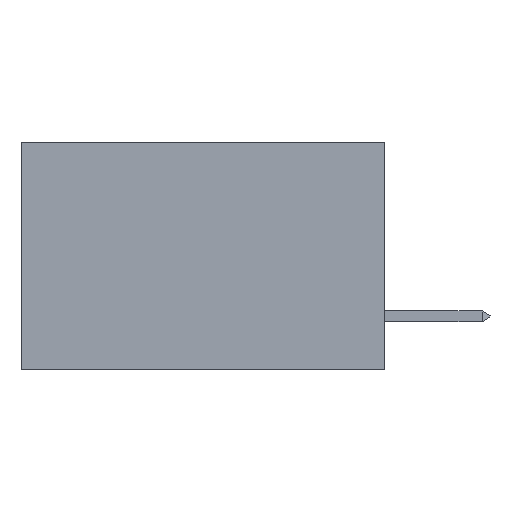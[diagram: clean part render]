
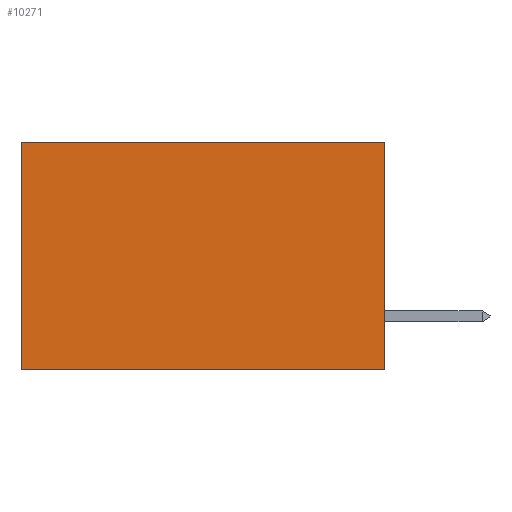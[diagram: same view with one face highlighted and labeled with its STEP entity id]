
A CAD part, left-side view. The second image highlights one B-rep face of the part: STEP entity #10271.
In plain terms, the highlighted planar face has unit normal (-1, 0, 0).
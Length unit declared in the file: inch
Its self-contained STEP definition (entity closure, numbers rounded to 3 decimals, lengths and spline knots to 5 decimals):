
#9 = VECTOR ( 'NONE', #11550, 39.37008 ) ;
#167 = DIRECTION ( 'NONE',  ( 1., 0., 0. ) ) ;
#1099 = AXIS2_PLACEMENT_3D ( 'NONE', #14096, #167, #14027 ) ;
#1627 = CARTESIAN_POINT ( 'NONE',  ( 0.2875, 0., -0.375 ) ) ;
#3702 = EDGE_CURVE ( 'NONE', #12875, #6642, #11055, .T. ) ;
#4436 = PLANE ( 'NONE',  #1099 ) ;
#5596 = CARTESIAN_POINT ( 'NONE',  ( 0.2875, 0.6, 0. ) ) ;
#5599 = LINE ( 'NONE', #14224, #12664 ) ;
#6515 = CARTESIAN_POINT ( 'NONE',  ( 0.2875, 0.6, -0.375 ) ) ;
#6580 = CARTESIAN_POINT ( 'NONE',  ( 0.2875, 0.6, -0.375 ) ) ;
#6642 = VERTEX_POINT ( 'NONE', #5596 ) ;
#7255 = ORIENTED_EDGE ( 'NONE', *, *, #12649, .F. ) ;
#7538 = VERTEX_POINT ( 'NONE', #1627 ) ;
#7686 = CARTESIAN_POINT ( 'NONE',  ( 0.2875, 0., 0. ) ) ;
#8364 = VERTEX_POINT ( 'NONE', #6580 ) ;
#8438 = EDGE_CURVE ( 'NONE', #6642, #8364, #12751, .T. ) ;
#9374 = CARTESIAN_POINT ( 'NONE',  ( 0.2875, 0., 0. ) ) ;
#9626 = EDGE_LOOP ( 'NONE', ( #13773, #7255, #12810, #14415 ) ) ;
#10271 = ADVANCED_FACE ( 'NONE', ( #15591 ), #4436, .F. ) ;
#11055 = LINE ( 'NONE', #9374, #15131 ) ;
#11550 = DIRECTION ( 'NONE',  ( 0., 1., 0. ) ) ;
#11990 = DIRECTION ( 'NONE',  ( 0., 1., 0. ) ) ;
#12649 = EDGE_CURVE ( 'NONE', #7538, #8364, #16769, .T. ) ;
#12664 = VECTOR ( 'NONE', #14164, 39.37008 ) ;
#12751 = LINE ( 'NONE', #6515, #13849 ) ;
#12810 = ORIENTED_EDGE ( 'NONE', *, *, #13257, .F. ) ;
#12875 = VERTEX_POINT ( 'NONE', #7686 ) ;
#13257 = EDGE_CURVE ( 'NONE', #12875, #7538, #5599, .T. ) ;
#13773 = ORIENTED_EDGE ( 'NONE', *, *, #8438, .T. ) ;
#13849 = VECTOR ( 'NONE', #16125, 39.37008 ) ;
#14027 = DIRECTION ( 'NONE',  ( 0., 0., -1. ) ) ;
#14096 = CARTESIAN_POINT ( 'NONE',  ( 0.2875, 0., -0.375 ) ) ;
#14164 = DIRECTION ( 'NONE',  ( 0., 0., -1. ) ) ;
#14224 = CARTESIAN_POINT ( 'NONE',  ( 0.2875, 0., -0.375 ) ) ;
#14415 = ORIENTED_EDGE ( 'NONE', *, *, #3702, .T. ) ;
#15131 = VECTOR ( 'NONE', #11990, 39.37008 ) ;
#15591 = FACE_OUTER_BOUND ( 'NONE', #9626, .T. ) ;
#16125 = DIRECTION ( 'NONE',  ( 0., 0., -1. ) ) ;
#16769 = LINE ( 'NONE', #17017, #9 ) ;
#17017 = CARTESIAN_POINT ( 'NONE',  ( 0.2875, 0., -0.375 ) ) ;
